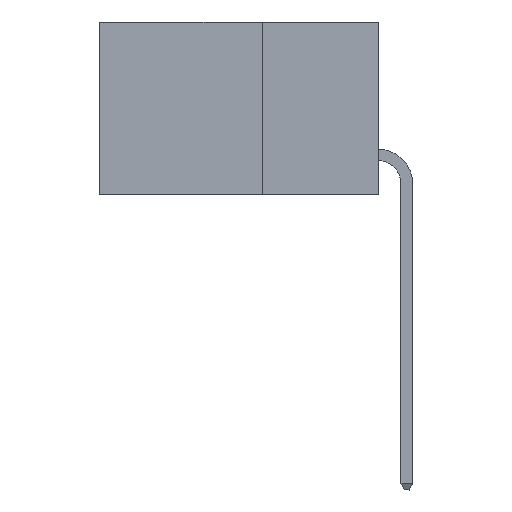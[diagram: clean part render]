
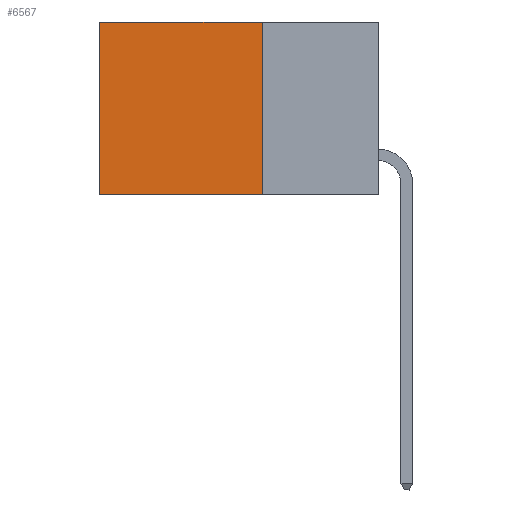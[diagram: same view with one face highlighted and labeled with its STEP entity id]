
A CAD part, left-side view. The second image highlights one B-rep face of the part: STEP entity #6567.
In plain terms, the highlighted planar face has unit normal (-1, 0, 0).
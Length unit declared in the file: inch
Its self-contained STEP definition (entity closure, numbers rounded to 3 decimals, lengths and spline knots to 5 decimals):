
#296 = ORIENTED_EDGE ( 'NONE', *, *, #16529, .T. ) ;
#1309 = CARTESIAN_POINT ( 'NONE',  ( 0.298, 0.25, 0. ) ) ;
#1911 = CARTESIAN_POINT ( 'NONE',  ( 0.298, 0.6, 0. ) ) ;
#3156 = DIRECTION ( 'NONE',  ( 0., 0., -1. ) ) ;
#3199 = EDGE_CURVE ( 'NONE', #8010, #4081, #6981, .T. ) ;
#3667 = EDGE_CURVE ( 'NONE', #10028, #22501, #15722, .T. ) ;
#4081 = VERTEX_POINT ( 'NONE', #13671 ) ;
#5398 = ORIENTED_EDGE ( 'NONE', *, *, #3667, .T. ) ;
#5621 = CARTESIAN_POINT ( 'NONE',  ( 0.298, 0.25, 0. ) ) ;
#5853 = EDGE_LOOP ( 'NONE', ( #5398, #12049, #8746, #296 ) ) ;
#6406 = VECTOR ( 'NONE', #22307, 39.37008 ) ;
#6567 = ADVANCED_FACE ( 'NONE', ( #9904 ), #12421, .F. ) ;
#6981 = LINE ( 'NONE', #16794, #11385 ) ;
#8010 = VERTEX_POINT ( 'NONE', #10986 ) ;
#8693 = CARTESIAN_POINT ( 'NONE',  ( 0.298, 0.6, 0. ) ) ;
#8746 = ORIENTED_EDGE ( 'NONE', *, *, #3199, .F. ) ;
#9904 = FACE_OUTER_BOUND ( 'NONE', #5853, .T. ) ;
#10028 = VERTEX_POINT ( 'NONE', #1911 ) ;
#10986 = CARTESIAN_POINT ( 'NONE',  ( 0.298, 0.25, 0. ) ) ;
#11385 = VECTOR ( 'NONE', #16823, 39.37008 ) ;
#11387 = LINE ( 'NONE', #5621, #6406 ) ;
#12049 = ORIENTED_EDGE ( 'NONE', *, *, #23292, .F. ) ;
#12421 = PLANE ( 'NONE',  #23610 ) ;
#12804 = VECTOR ( 'NONE', #18003, 39.37008 ) ;
#13671 = CARTESIAN_POINT ( 'NONE',  ( 0.298, 0.25, -0.37 ) ) ;
#14313 = DIRECTION ( 'NONE',  ( 1., 0., 0. ) ) ;
#14420 = DIRECTION ( 'NONE',  ( 0., 0., -1. ) ) ;
#15153 = VECTOR ( 'NONE', #14420, 39.37008 ) ;
#15722 = LINE ( 'NONE', #8693, #15153 ) ;
#16529 = EDGE_CURVE ( 'NONE', #8010, #10028, #11387, .T. ) ;
#16794 = CARTESIAN_POINT ( 'NONE',  ( 0.298, 0.25, 0. ) ) ;
#16823 = DIRECTION ( 'NONE',  ( 0., 0., -1. ) ) ;
#18003 = DIRECTION ( 'NONE',  ( 0., 1., 0. ) ) ;
#21550 = CARTESIAN_POINT ( 'NONE',  ( 0.298, 0.6, -0.37 ) ) ;
#21594 = CARTESIAN_POINT ( 'NONE',  ( 0.298, 0.25, -0.37 ) ) ;
#22307 = DIRECTION ( 'NONE',  ( 0., 1., 0. ) ) ;
#22501 = VERTEX_POINT ( 'NONE', #21550 ) ;
#22626 = LINE ( 'NONE', #21594, #12804 ) ;
#23292 = EDGE_CURVE ( 'NONE', #4081, #22501, #22626, .T. ) ;
#23610 = AXIS2_PLACEMENT_3D ( 'NONE', #1309, #14313, #3156 ) ;
